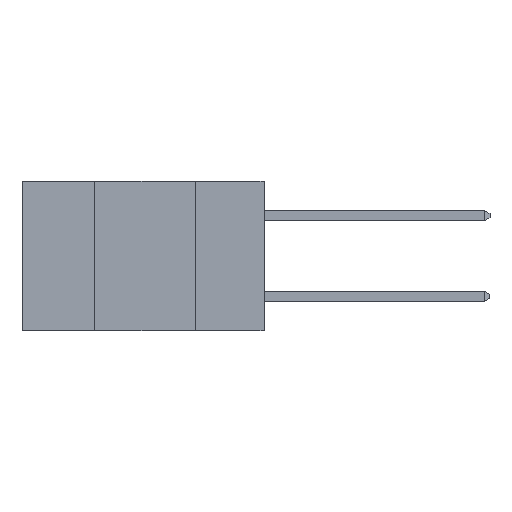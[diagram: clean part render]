
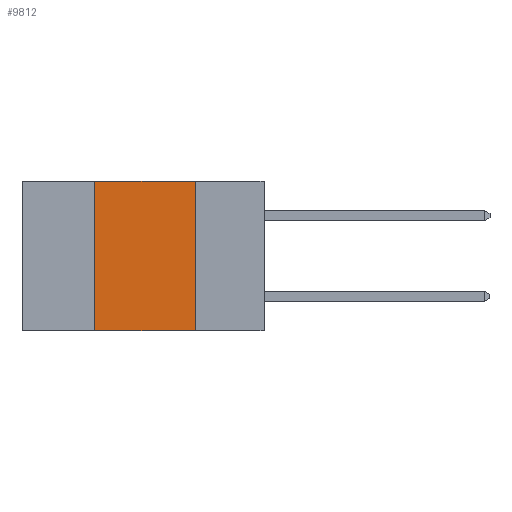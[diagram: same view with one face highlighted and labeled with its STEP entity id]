
A CAD part, left-side view. The second image highlights one B-rep face of the part: STEP entity #9812.
In plain terms, the highlighted planar face has unit normal (-1, 0, 0).
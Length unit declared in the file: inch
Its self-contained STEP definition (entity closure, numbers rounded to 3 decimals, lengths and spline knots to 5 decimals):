
#615 = ORIENTED_EDGE ( 'NONE', *, *, #2076, .F. ) ;
#683 = DIRECTION ( 'NONE',  ( 0., 0., -1. ) ) ;
#723 = DIRECTION ( 'NONE',  ( 0., -1., 0. ) ) ;
#1878 = CARTESIAN_POINT ( 'NONE',  ( 0., 0.17, -0.37 ) ) ;
#1934 = EDGE_CURVE ( 'NONE', #12763, #16887, #6766, .T. ) ;
#1992 = VECTOR ( 'NONE', #10483, 39.37008 ) ;
#2076 = EDGE_CURVE ( 'NONE', #12318, #5651, #15490, .T. ) ;
#3359 = CARTESIAN_POINT ( 'NONE',  ( 0., 0.42, 0. ) ) ;
#3409 = CARTESIAN_POINT ( 'NONE',  ( 0., 0.17, 0. ) ) ;
#4202 = CARTESIAN_POINT ( 'NONE',  ( 0., 0.17, 0. ) ) ;
#4548 = EDGE_LOOP ( 'NONE', ( #12035, #615, #8272, #15188 ) ) ;
#4851 = DIRECTION ( 'NONE',  ( 0., 0., -1. ) ) ;
#5583 = LINE ( 'NONE', #3409, #12776 ) ;
#5651 = VERTEX_POINT ( 'NONE', #4202 ) ;
#6766 = LINE ( 'NONE', #13133, #10121 ) ;
#7905 = VECTOR ( 'NONE', #12409, 39.37008 ) ;
#8089 = CARTESIAN_POINT ( 'NONE',  ( 0., 0.42, -0.37 ) ) ;
#8272 = ORIENTED_EDGE ( 'NONE', *, *, #12493, .F. ) ;
#9276 = DIRECTION ( 'NONE',  ( 1., 0., 0. ) ) ;
#9611 = LINE ( 'NONE', #3359, #1992 ) ;
#9812 = ADVANCED_FACE ( 'NONE', ( #12835 ), #17818, .F. ) ;
#10121 = VECTOR ( 'NONE', #723, 39.37008 ) ;
#10123 = CARTESIAN_POINT ( 'NONE',  ( 0., 0.42, 0. ) ) ;
#10483 = DIRECTION ( 'NONE',  ( 0., 0., 1. ) ) ;
#11170 = EDGE_CURVE ( 'NONE', #5651, #16887, #5583, .T. ) ;
#11595 = AXIS2_PLACEMENT_3D ( 'NONE', #12094, #9276, #683 ) ;
#12035 = ORIENTED_EDGE ( 'NONE', *, *, #11170, .F. ) ;
#12094 = CARTESIAN_POINT ( 'NONE',  ( 0., 0.6, 0. ) ) ;
#12318 = VERTEX_POINT ( 'NONE', #10123 ) ;
#12409 = DIRECTION ( 'NONE',  ( 0., -1., 0. ) ) ;
#12493 = EDGE_CURVE ( 'NONE', #12763, #12318, #9611, .T. ) ;
#12763 = VERTEX_POINT ( 'NONE', #8089 ) ;
#12776 = VECTOR ( 'NONE', #4851, 39.37008 ) ;
#12835 = FACE_OUTER_BOUND ( 'NONE', #4548, .T. ) ;
#13133 = CARTESIAN_POINT ( 'NONE',  ( 0., 0.6, -0.37 ) ) ;
#14061 = CARTESIAN_POINT ( 'NONE',  ( 0., 0.6, 0. ) ) ;
#15188 = ORIENTED_EDGE ( 'NONE', *, *, #1934, .T. ) ;
#15490 = LINE ( 'NONE', #14061, #7905 ) ;
#16887 = VERTEX_POINT ( 'NONE', #1878 ) ;
#17818 = PLANE ( 'NONE',  #11595 ) ;
